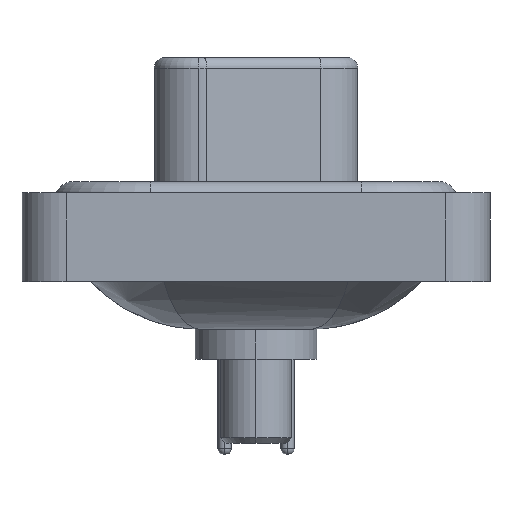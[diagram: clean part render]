
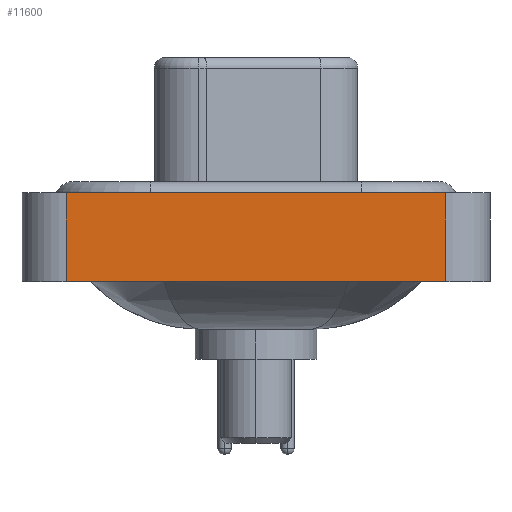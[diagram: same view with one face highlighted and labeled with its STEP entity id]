
A CAD part, left-side view. The second image highlights one B-rep face of the part: STEP entity #11600.
In plain terms, the highlighted planar face has unit normal (-1, 0, 0).
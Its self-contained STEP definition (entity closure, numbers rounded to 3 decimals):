
#323 = CARTESIAN_POINT ( 'NONE',  ( -7.3, -8.55, -3.6 ) ) ;
#1056 = LINE ( 'NONE', #17619, #12903 ) ;
#2546 = CARTESIAN_POINT ( 'NONE',  ( -7.3, 8.55, -3.6 ) ) ;
#3250 = CARTESIAN_POINT ( 'NONE',  ( -7.3, -8.55, 0.4 ) ) ;
#3885 = VERTEX_POINT ( 'NONE', #3250 ) ;
#4189 = EDGE_CURVE ( 'NONE', #5745, #12357, #1056, .T. ) ;
#4543 = LINE ( 'NONE', #10379, #10753 ) ;
#4964 = LINE ( 'NONE', #12685, #17193 ) ;
#5745 = VERTEX_POINT ( 'NONE', #2546 ) ;
#6342 = DIRECTION ( 'NONE',  ( -1., 0., 0. ) ) ;
#6376 = ORIENTED_EDGE ( 'NONE', *, *, #15116, .F. ) ;
#7836 = FACE_OUTER_BOUND ( 'NONE', #18025, .T. ) ;
#7984 = EDGE_CURVE ( 'NONE', #10043, #3885, #4964, .T. ) ;
#8765 = DIRECTION ( 'NONE',  ( 0., -1., 0. ) ) ;
#9376 = ORIENTED_EDGE ( 'NONE', *, *, #7984, .F. ) ;
#9557 = ORIENTED_EDGE ( 'NONE', *, *, #15231, .T. ) ;
#10043 = VERTEX_POINT ( 'NONE', #13674 ) ;
#10379 = CARTESIAN_POINT ( 'NONE',  ( -7.3, -8.55, -3.6 ) ) ;
#10753 = VECTOR ( 'NONE', #17860, 1000. ) ;
#11091 = AXIS2_PLACEMENT_3D ( 'NONE', #323, #6342, #12395 ) ;
#11269 = ORIENTED_EDGE ( 'NONE', *, *, #4189, .T. ) ;
#11567 = LINE ( 'NONE', #13061, #17349 ) ;
#11600 = ADVANCED_FACE ( 'NONE', ( #7836 ), #13858, .T. ) ;
#12357 = VERTEX_POINT ( 'NONE', #13883 ) ;
#12395 = DIRECTION ( 'NONE',  ( 0., 0., 1. ) ) ;
#12685 = CARTESIAN_POINT ( 'NONE',  ( -7.3, -8.55, 0.4 ) ) ;
#12903 = VECTOR ( 'NONE', #8765, 1000. ) ;
#13061 = CARTESIAN_POINT ( 'NONE',  ( -7.3, 8.55, -3.6 ) ) ;
#13674 = CARTESIAN_POINT ( 'NONE',  ( -7.3, 8.55, 0.4 ) ) ;
#13858 = PLANE ( 'NONE',  #11091 ) ;
#13883 = CARTESIAN_POINT ( 'NONE',  ( -7.3, -8.55, -3.6 ) ) ;
#15116 = EDGE_CURVE ( 'NONE', #5745, #10043, #11567, .T. ) ;
#15231 = EDGE_CURVE ( 'NONE', #12357, #3885, #4543, .T. ) ;
#16990 = DIRECTION ( 'NONE',  ( 0., -1., 0. ) ) ;
#17193 = VECTOR ( 'NONE', #16990, 1000. ) ;
#17349 = VECTOR ( 'NONE', #17563, 1000. ) ;
#17563 = DIRECTION ( 'NONE',  ( 0., 0., 1. ) ) ;
#17619 = CARTESIAN_POINT ( 'NONE',  ( -7.3, -8.55, -3.6 ) ) ;
#17860 = DIRECTION ( 'NONE',  ( 0., 0., 1. ) ) ;
#18025 = EDGE_LOOP ( 'NONE', ( #9557, #9376, #6376, #11269 ) ) ;
